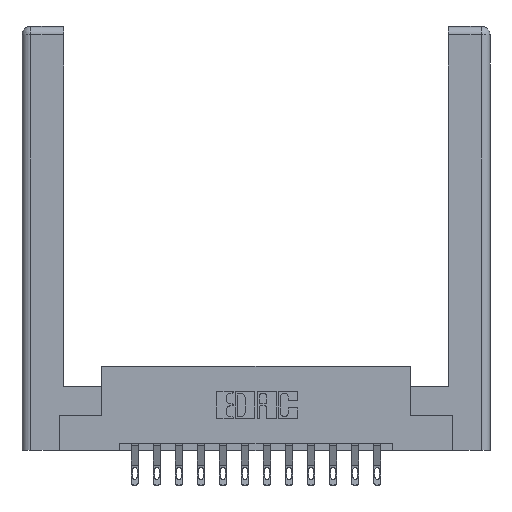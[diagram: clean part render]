
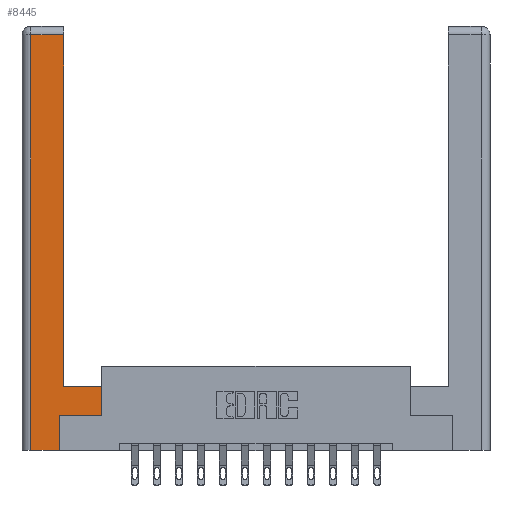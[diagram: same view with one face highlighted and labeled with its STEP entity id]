
A CAD part, top view. The second image highlights one B-rep face of the part: STEP entity #8445.
In plain terms, the highlighted planar face has unit normal (0, 0, 1).
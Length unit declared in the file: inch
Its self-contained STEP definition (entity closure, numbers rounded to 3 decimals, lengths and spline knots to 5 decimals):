
#606 = ORIENTED_EDGE ( 'NONE', *, *, #12348, .T. ) ;
#865 = DIRECTION ( 'NONE',  ( 0., 1., 0. ) ) ;
#956 = LINE ( 'NONE', #14826, #13875 ) ;
#993 = VECTOR ( 'NONE', #13184, 39.37008 ) ;
#999 = VERTEX_POINT ( 'NONE', #11375 ) ;
#1005 = CARTESIAN_POINT ( 'NONE',  ( 0.265, 0., 0. ) ) ;
#1049 = EDGE_CURVE ( 'NONE', #12948, #9267, #11778, .T. ) ;
#1775 = CARTESIAN_POINT ( 'NONE',  ( 0.0615, 0., 0. ) ) ;
#2258 = CARTESIAN_POINT ( 'NONE',  ( 0.565, 0.245, 0. ) ) ;
#2612 = ORIENTED_EDGE ( 'NONE', *, *, #4774, .T. ) ;
#3263 = CARTESIAN_POINT ( 'NONE',  ( 0., 0., 0. ) ) ;
#3514 = EDGE_CURVE ( 'NONE', #10053, #12948, #956, .T. ) ;
#4031 = VECTOR ( 'NONE', #5671, 39.37008 ) ;
#4371 = DIRECTION ( 'NONE',  ( 0., 0., -1. ) ) ;
#4574 = CARTESIAN_POINT ( 'NONE',  ( 0.265, 0., 0. ) ) ;
#4658 = LINE ( 'NONE', #14338, #11097 ) ;
#4774 = EDGE_CURVE ( 'NONE', #12639, #10053, #8370, .T. ) ;
#5053 = CARTESIAN_POINT ( 'NONE',  ( 0.295, 0.45, 0. ) ) ;
#5628 = EDGE_CURVE ( 'NONE', #9267, #14964, #7174, .T. ) ;
#5671 = DIRECTION ( 'NONE',  ( 1., 0., 0. ) ) ;
#5712 = DIRECTION ( 'NONE',  ( -1., 0., 0. ) ) ;
#5805 = ORIENTED_EDGE ( 'NONE', *, *, #1049, .T. ) ;
#6268 = CARTESIAN_POINT ( 'NONE',  ( 0.295, 0.45, 0. ) ) ;
#6844 = AXIS2_PLACEMENT_3D ( 'NONE', #3263, #4371, #5712 ) ;
#7171 = EDGE_LOOP ( 'NONE', ( #9228, #606, #10639, #9943, #2612, #11112, #5805, #8446 ) ) ;
#7174 = LINE ( 'NONE', #6268, #7952 ) ;
#7257 = DIRECTION ( 'NONE',  ( -1., 0., 0. ) ) ;
#7952 = VECTOR ( 'NONE', #7257, 39.37008 ) ;
#8370 = LINE ( 'NONE', #10033, #9323 ) ;
#8445 = ADVANCED_FACE ( 'NONE', ( #12730 ), #14433, .F. ) ;
#8446 = ORIENTED_EDGE ( 'NONE', *, *, #5628, .T. ) ;
#8450 = VECTOR ( 'NONE', #865, 39.37008 ) ;
#9027 = EDGE_CURVE ( 'NONE', #999, #9588, #14287, .T. ) ;
#9228 = ORIENTED_EDGE ( 'NONE', *, *, #12363, .T. ) ;
#9267 = VERTEX_POINT ( 'NONE', #13554 ) ;
#9323 = VECTOR ( 'NONE', #10205, 39.37008 ) ;
#9588 = VERTEX_POINT ( 'NONE', #1775 ) ;
#9943 = ORIENTED_EDGE ( 'NONE', *, *, #14203, .T. ) ;
#10033 = CARTESIAN_POINT ( 'NONE',  ( 0.265, 0.245, 0. ) ) ;
#10043 = LINE ( 'NONE', #4574, #4031 ) ;
#10053 = VERTEX_POINT ( 'NONE', #12815 ) ;
#10086 = DIRECTION ( 'NONE',  ( 1., 0., 0. ) ) ;
#10205 = DIRECTION ( 'NONE',  ( 0., 1., 0. ) ) ;
#10639 = ORIENTED_EDGE ( 'NONE', *, *, #9027, .T. ) ;
#10884 = CARTESIAN_POINT ( 'NONE',  ( 0.0615, 0., 0. ) ) ;
#10985 = CARTESIAN_POINT ( 'NONE',  ( 0.565, 0.45, 0. ) ) ;
#11097 = VECTOR ( 'NONE', #13054, 39.37008 ) ;
#11112 = ORIENTED_EDGE ( 'NONE', *, *, #3514, .T. ) ;
#11375 = CARTESIAN_POINT ( 'NONE',  ( 0.0615, 2.94, 0. ) ) ;
#11778 = LINE ( 'NONE', #10985, #8450 ) ;
#12348 = EDGE_CURVE ( 'NONE', #15009, #999, #4658, .T. ) ;
#12363 = EDGE_CURVE ( 'NONE', #14964, #15009, #16153, .T. ) ;
#12639 = VERTEX_POINT ( 'NONE', #1005 ) ;
#12676 = VECTOR ( 'NONE', #14126, 39.37008 ) ;
#12730 = FACE_OUTER_BOUND ( 'NONE', #7171, .T. ) ;
#12815 = CARTESIAN_POINT ( 'NONE',  ( 0.265, 0.245, 0. ) ) ;
#12948 = VERTEX_POINT ( 'NONE', #2258 ) ;
#13054 = DIRECTION ( 'NONE',  ( -1., 0., 0. ) ) ;
#13184 = DIRECTION ( 'NONE',  ( 0., -1., 0. ) ) ;
#13554 = CARTESIAN_POINT ( 'NONE',  ( 0.565, 0.45, 0. ) ) ;
#13574 = CARTESIAN_POINT ( 'NONE',  ( 0.295, 2.94, 0. ) ) ;
#13875 = VECTOR ( 'NONE', #10086, 39.37008 ) ;
#14126 = DIRECTION ( 'NONE',  ( 0., 1., 0. ) ) ;
#14203 = EDGE_CURVE ( 'NONE', #9588, #12639, #10043, .T. ) ;
#14287 = LINE ( 'NONE', #10884, #993 ) ;
#14338 = CARTESIAN_POINT ( 'NONE',  ( 0.0615, 2.94, 0. ) ) ;
#14433 = PLANE ( 'NONE',  #6844 ) ;
#14826 = CARTESIAN_POINT ( 'NONE',  ( 0.565, 0.245, 0. ) ) ;
#14964 = VERTEX_POINT ( 'NONE', #5053 ) ;
#15009 = VERTEX_POINT ( 'NONE', #13574 ) ;
#15425 = CARTESIAN_POINT ( 'NONE',  ( 0.295, 3., 0. ) ) ;
#16153 = LINE ( 'NONE', #15425, #12676 ) ;
